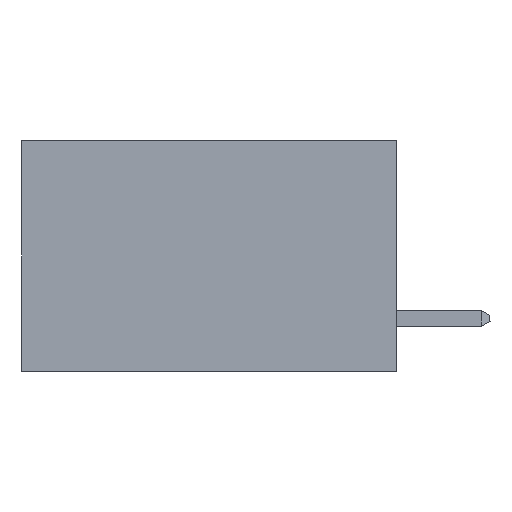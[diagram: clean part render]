
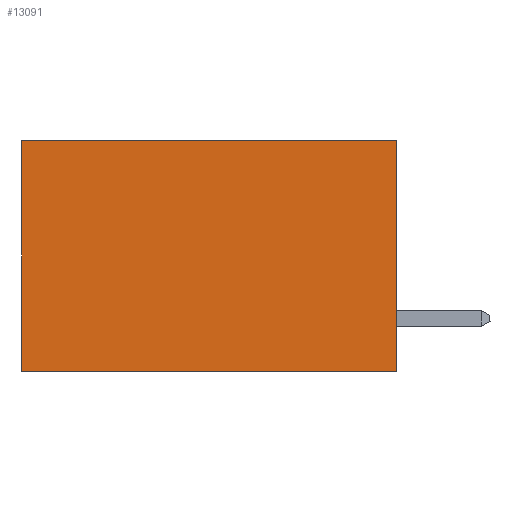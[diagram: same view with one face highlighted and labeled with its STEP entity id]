
A CAD part, left-side view. The second image highlights one B-rep face of the part: STEP entity #13091.
In plain terms, the highlighted planar face has unit normal (-1, 0, 0).
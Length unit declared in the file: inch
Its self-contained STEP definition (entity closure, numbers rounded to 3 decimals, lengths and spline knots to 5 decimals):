
#37 = VECTOR ( 'NONE', #13912, 39.37008 ) ;
#1057 = FACE_OUTER_BOUND ( 'NONE', #15998, .T. ) ;
#1260 = CARTESIAN_POINT ( 'NONE',  ( 0.298, 0., 0. ) ) ;
#1508 = AXIS2_PLACEMENT_3D ( 'NONE', #1260, #2776, #13324 ) ;
#1609 = CARTESIAN_POINT ( 'NONE',  ( 0.298, 0., -0.37 ) ) ;
#2776 = DIRECTION ( 'NONE',  ( 1., 0., 0. ) ) ;
#4149 = EDGE_CURVE ( 'NONE', #13246, #18327, #8076, .T. ) ;
#4647 = EDGE_CURVE ( 'NONE', #5952, #13246, #7583, .T. ) ;
#4832 = DIRECTION ( 'NONE',  ( 0., 0., -1. ) ) ;
#4840 = DIRECTION ( 'NONE',  ( 0., 1., 0. ) ) ;
#5040 = ORIENTED_EDGE ( 'NONE', *, *, #16330, .T. ) ;
#5952 = VERTEX_POINT ( 'NONE', #13583 ) ;
#7005 = CARTESIAN_POINT ( 'NONE',  ( 0.298, 0.6, -0.37 ) ) ;
#7164 = LINE ( 'NONE', #18260, #15057 ) ;
#7583 = LINE ( 'NONE', #11551, #14570 ) ;
#7847 = CARTESIAN_POINT ( 'NONE',  ( 0.298, 0., 0. ) ) ;
#8076 = LINE ( 'NONE', #13908, #37 ) ;
#8117 = VERTEX_POINT ( 'NONE', #11660 ) ;
#8822 = ORIENTED_EDGE ( 'NONE', *, *, #8954, .T. ) ;
#8954 = EDGE_CURVE ( 'NONE', #8117, #18327, #7164, .T. ) ;
#10352 = PLANE ( 'NONE',  #1508 ) ;
#10755 = ORIENTED_EDGE ( 'NONE', *, *, #4149, .F. ) ;
#10857 = DIRECTION ( 'NONE',  ( 0., 0., -1. ) ) ;
#11551 = CARTESIAN_POINT ( 'NONE',  ( 0.298, 0., 0. ) ) ;
#11660 = CARTESIAN_POINT ( 'NONE',  ( 0.298, 0.6, 0. ) ) ;
#11929 = LINE ( 'NONE', #7847, #18786 ) ;
#13091 = ADVANCED_FACE ( 'NONE', ( #1057 ), #10352, .F. ) ;
#13246 = VERTEX_POINT ( 'NONE', #1609 ) ;
#13324 = DIRECTION ( 'NONE',  ( 0., 0., -1. ) ) ;
#13338 = ORIENTED_EDGE ( 'NONE', *, *, #4647, .F. ) ;
#13583 = CARTESIAN_POINT ( 'NONE',  ( 0.298, 0., 0. ) ) ;
#13908 = CARTESIAN_POINT ( 'NONE',  ( 0.298, 0., -0.37 ) ) ;
#13912 = DIRECTION ( 'NONE',  ( 0., 1., 0. ) ) ;
#14570 = VECTOR ( 'NONE', #10857, 39.37008 ) ;
#15057 = VECTOR ( 'NONE', #4832, 39.37008 ) ;
#15998 = EDGE_LOOP ( 'NONE', ( #8822, #10755, #13338, #5040 ) ) ;
#16330 = EDGE_CURVE ( 'NONE', #5952, #8117, #11929, .T. ) ;
#18260 = CARTESIAN_POINT ( 'NONE',  ( 0.298, 0.6, 0. ) ) ;
#18327 = VERTEX_POINT ( 'NONE', #7005 ) ;
#18786 = VECTOR ( 'NONE', #4840, 39.37008 ) ;
